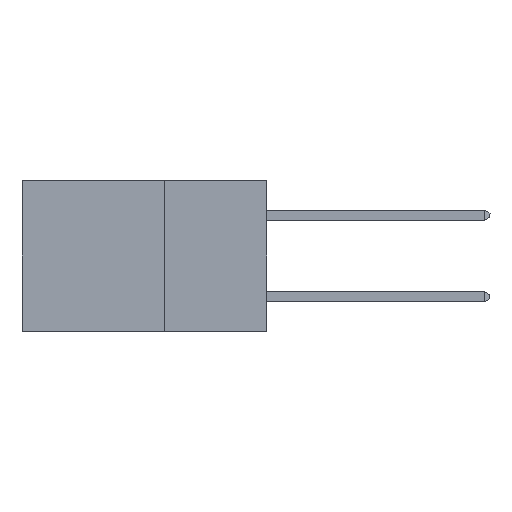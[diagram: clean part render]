
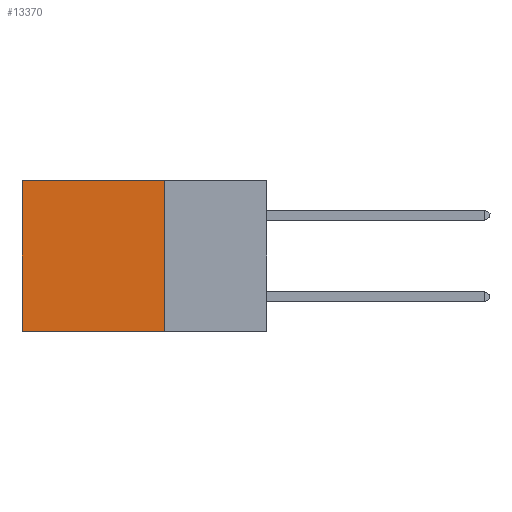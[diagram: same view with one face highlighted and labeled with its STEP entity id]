
A CAD part, left-side view. The second image highlights one B-rep face of the part: STEP entity #13370.
In plain terms, the highlighted planar face has unit normal (-1, 0, 0).
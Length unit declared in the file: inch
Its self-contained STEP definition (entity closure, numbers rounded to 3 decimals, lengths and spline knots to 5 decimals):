
#61 = CARTESIAN_POINT ( 'NONE',  ( 0.2875, 0.6, -0.37 ) ) ;
#1602 = ORIENTED_EDGE ( 'NONE', *, *, #5184, .F. ) ;
#3563 = DIRECTION ( 'NONE',  ( 0., 1., 0. ) ) ;
#3564 = LINE ( 'NONE', #9883, #11304 ) ;
#4573 = LINE ( 'NONE', #5170, #12256 ) ;
#5170 = CARTESIAN_POINT ( 'NONE',  ( 0.2875, 0.25, -0.37 ) ) ;
#5184 = EDGE_CURVE ( 'NONE', #16107, #15590, #4573, .T. ) ;
#5239 = EDGE_CURVE ( 'NONE', #12011, #16107, #3564, .T. ) ;
#5250 = VECTOR ( 'NONE', #19228, 39.37008 ) ;
#5713 = LINE ( 'NONE', #17734, #5250 ) ;
#6080 = CARTESIAN_POINT ( 'NONE',  ( 0.2875, 0.25, 0. ) ) ;
#6147 = PLANE ( 'NONE',  #19694 ) ;
#6728 = CARTESIAN_POINT ( 'NONE',  ( 0.2875, 0.6, 0. ) ) ;
#7160 = ORIENTED_EDGE ( 'NONE', *, *, #5239, .F. ) ;
#7501 = CARTESIAN_POINT ( 'NONE',  ( 0.2875, 0.25, -0.37 ) ) ;
#7511 = CARTESIAN_POINT ( 'NONE',  ( 0.2875, 0.6, 0. ) ) ;
#7700 = DIRECTION ( 'NONE',  ( 1., 0., 0. ) ) ;
#9195 = VECTOR ( 'NONE', #19601, 39.37008 ) ;
#9883 = CARTESIAN_POINT ( 'NONE',  ( 0.2875, 0.25, 0. ) ) ;
#10838 = EDGE_CURVE ( 'NONE', #12413, #15590, #17213, .T. ) ;
#11304 = VECTOR ( 'NONE', #11402, 39.37008 ) ;
#11402 = DIRECTION ( 'NONE',  ( 0., 0., -1. ) ) ;
#12011 = VERTEX_POINT ( 'NONE', #16429 ) ;
#12129 = ORIENTED_EDGE ( 'NONE', *, *, #10838, .T. ) ;
#12256 = VECTOR ( 'NONE', #3563, 39.37008 ) ;
#12413 = VERTEX_POINT ( 'NONE', #6728 ) ;
#12869 = ORIENTED_EDGE ( 'NONE', *, *, #13443, .T. ) ;
#13370 = ADVANCED_FACE ( 'NONE', ( #18775 ), #6147, .F. ) ;
#13443 = EDGE_CURVE ( 'NONE', #12011, #12413, #5713, .T. ) ;
#15590 = VERTEX_POINT ( 'NONE', #61 ) ;
#16107 = VERTEX_POINT ( 'NONE', #7501 ) ;
#16429 = CARTESIAN_POINT ( 'NONE',  ( 0.2875, 0.25, 0. ) ) ;
#17213 = LINE ( 'NONE', #7511, #9195 ) ;
#17734 = CARTESIAN_POINT ( 'NONE',  ( 0.2875, 0.25, 0. ) ) ;
#18287 = DIRECTION ( 'NONE',  ( 0., 0., -1. ) ) ;
#18775 = FACE_OUTER_BOUND ( 'NONE', #19628, .T. ) ;
#19228 = DIRECTION ( 'NONE',  ( 0., 1., 0. ) ) ;
#19601 = DIRECTION ( 'NONE',  ( 0., 0., -1. ) ) ;
#19628 = EDGE_LOOP ( 'NONE', ( #12129, #1602, #7160, #12869 ) ) ;
#19694 = AXIS2_PLACEMENT_3D ( 'NONE', #6080, #7700, #18287 ) ;
